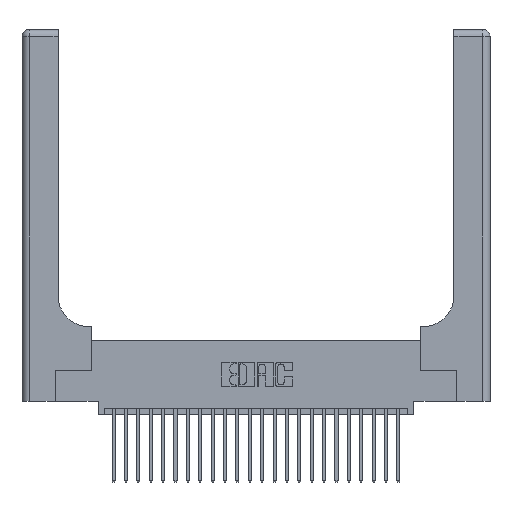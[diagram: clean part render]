
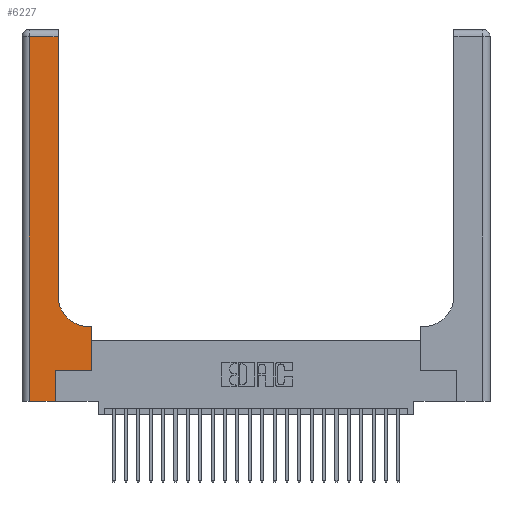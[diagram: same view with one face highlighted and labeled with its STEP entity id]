
A CAD part, top view. The second image highlights one B-rep face of the part: STEP entity #6227.
In plain terms, the highlighted planar face has unit normal (0, 0, 1).
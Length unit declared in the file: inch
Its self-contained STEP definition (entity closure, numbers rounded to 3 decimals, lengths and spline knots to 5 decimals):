
#81 = VECTOR ( 'NONE', #18370, 39.37008 ) ;
#150 = CARTESIAN_POINT ( 'NONE',  ( 0.06, 2.94, 0.37 ) ) ;
#1315 = DIRECTION ( 'NONE',  ( 0., 0., -1. ) ) ;
#1392 = VECTOR ( 'NONE', #13062, 39.37008 ) ;
#1526 = DIRECTION ( 'NONE',  ( 0., 0., -1. ) ) ;
#1726 = VECTOR ( 'NONE', #19725, 39.37008 ) ;
#2186 = VECTOR ( 'NONE', #19646, 39.37008 ) ;
#2358 = VERTEX_POINT ( 'NONE', #21892 ) ;
#2369 = VECTOR ( 'NONE', #26417, 39.37008 ) ;
#3182 = CARTESIAN_POINT ( 'NONE',  ( 0.06, 3., 0.37 ) ) ;
#3226 = ORIENTED_EDGE ( 'NONE', *, *, #23611, .T. ) ;
#3460 = DIRECTION ( 'NONE',  ( 0., 1., 0. ) ) ;
#3905 = VERTEX_POINT ( 'NONE', #8885 ) ;
#5863 = VECTOR ( 'NONE', #3460, 39.37008 ) ;
#5984 = ORIENTED_EDGE ( 'NONE', *, *, #18857, .T. ) ;
#6227 = ADVANCED_FACE ( 'NONE', ( #16225 ), #24221, .F. ) ;
#6381 = LINE ( 'NONE', #25629, #2186 ) ;
#6566 = ORIENTED_EDGE ( 'NONE', *, *, #21321, .T. ) ;
#6861 = LINE ( 'NONE', #20578, #1392 ) ;
#7217 = CARTESIAN_POINT ( 'NONE',  ( 0., 0., 0.37 ) ) ;
#7303 = DIRECTION ( 'NONE',  ( 1., 0., 0. ) ) ;
#7667 = VERTEX_POINT ( 'NONE', #13501 ) ;
#7918 = ORIENTED_EDGE ( 'NONE', *, *, #23256, .T. ) ;
#7946 = EDGE_CURVE ( 'NONE', #7667, #3905, #6861, .T. ) ;
#8885 = CARTESIAN_POINT ( 'NONE',  ( 0.2915, 2.94, 0.37 ) ) ;
#9073 = ORIENTED_EDGE ( 'NONE', *, *, #24730, .T. ) ;
#9453 = CARTESIAN_POINT ( 'NONE',  ( 0.5585, 0.25, 0.37 ) ) ;
#9688 = CARTESIAN_POINT ( 'NONE',  ( 0., 3., 0.37 ) ) ;
#9750 = EDGE_LOOP ( 'NONE', ( #25004, #6566, #9073, #5984, #22125, #23562, #7918, #3226, #13375 ) ) ;
#9998 = LINE ( 'NONE', #11545, #5863 ) ;
#10092 = LINE ( 'NONE', #22646, #10747 ) ;
#10422 = CARTESIAN_POINT ( 'NONE',  ( 0.5585, 0.6, 0.37 ) ) ;
#10747 = VECTOR ( 'NONE', #18426, 39.37008 ) ;
#11545 = CARTESIAN_POINT ( 'NONE',  ( 0.5585, 0.25, 0.37 ) ) ;
#11564 = CARTESIAN_POINT ( 'NONE',  ( 0.5415, 0.85, 0.37 ) ) ;
#13010 = LINE ( 'NONE', #17922, #2369 ) ;
#13062 = DIRECTION ( 'NONE',  ( 0., 1., 0. ) ) ;
#13307 = LINE ( 'NONE', #3182, #1726 ) ;
#13317 = AXIS2_PLACEMENT_3D ( 'NONE', #9688, #1526, #25962 ) ;
#13375 = ORIENTED_EDGE ( 'NONE', *, *, #15625, .T. ) ;
#13501 = CARTESIAN_POINT ( 'NONE',  ( 0.2915, 0.85, 0.37 ) ) ;
#13927 = LINE ( 'NONE', #22666, #81 ) ;
#14265 = VECTOR ( 'NONE', #7303, 39.37008 ) ;
#14635 = EDGE_CURVE ( 'NONE', #26550, #23667, #13010, .T. ) ;
#14663 = AXIS2_PLACEMENT_3D ( 'NONE', #11564, #1315, #15711 ) ;
#15625 = EDGE_CURVE ( 'NONE', #2358, #7667, #23587, .T. ) ;
#15711 = DIRECTION ( 'NONE',  ( 1., 0., 0. ) ) ;
#15851 = EDGE_CURVE ( 'NONE', #23667, #21543, #13927, .T. ) ;
#16225 = FACE_OUTER_BOUND ( 'NONE', #9750, .T. ) ;
#16467 = VERTEX_POINT ( 'NONE', #150 ) ;
#17165 = LINE ( 'NONE', #7217, #14265 ) ;
#17922 = CARTESIAN_POINT ( 'NONE',  ( 0.269, 0., 0.37 ) ) ;
#18370 = DIRECTION ( 'NONE',  ( 1., 0., 0. ) ) ;
#18426 = DIRECTION ( 'NONE',  ( -1., 0., 0. ) ) ;
#18597 = CARTESIAN_POINT ( 'NONE',  ( 0.06, 0., 0.37 ) ) ;
#18857 = EDGE_CURVE ( 'NONE', #21773, #26550, #17165, .T. ) ;
#19646 = DIRECTION ( 'NONE',  ( -1., 0., 0. ) ) ;
#19725 = DIRECTION ( 'NONE',  ( 0., -1., 0. ) ) ;
#20578 = CARTESIAN_POINT ( 'NONE',  ( 0.2915, 3., 0.37 ) ) ;
#21321 = EDGE_CURVE ( 'NONE', #3905, #16467, #6381, .T. ) ;
#21543 = VERTEX_POINT ( 'NONE', #9453 ) ;
#21773 = VERTEX_POINT ( 'NONE', #18597 ) ;
#21892 = CARTESIAN_POINT ( 'NONE',  ( 0.5415, 0.6, 0.37 ) ) ;
#22125 = ORIENTED_EDGE ( 'NONE', *, *, #14635, .T. ) ;
#22646 = CARTESIAN_POINT ( 'NONE',  ( 0.2915, 0.6, 0.37 ) ) ;
#22666 = CARTESIAN_POINT ( 'NONE',  ( 0.269, 0.25, 0.37 ) ) ;
#22971 = VERTEX_POINT ( 'NONE', #10422 ) ;
#23256 = EDGE_CURVE ( 'NONE', #21543, #22971, #9998, .T. ) ;
#23562 = ORIENTED_EDGE ( 'NONE', *, *, #15851, .T. ) ;
#23587 = CIRCLE ( 'NONE', #14663, 0.25 ) ;
#23611 = EDGE_CURVE ( 'NONE', #22971, #2358, #10092, .T. ) ;
#23667 = VERTEX_POINT ( 'NONE', #24939 ) ;
#24221 = PLANE ( 'NONE',  #13317 ) ;
#24730 = EDGE_CURVE ( 'NONE', #16467, #21773, #13307, .T. ) ;
#24939 = CARTESIAN_POINT ( 'NONE',  ( 0.269, 0.25, 0.37 ) ) ;
#25004 = ORIENTED_EDGE ( 'NONE', *, *, #7946, .T. ) ;
#25629 = CARTESIAN_POINT ( 'NONE',  ( 0., 2.94, 0.37 ) ) ;
#25701 = CARTESIAN_POINT ( 'NONE',  ( 0.269, 0., 0.37 ) ) ;
#25962 = DIRECTION ( 'NONE',  ( -1., 0., 0. ) ) ;
#26417 = DIRECTION ( 'NONE',  ( 0., 1., 0. ) ) ;
#26550 = VERTEX_POINT ( 'NONE', #25701 ) ;
